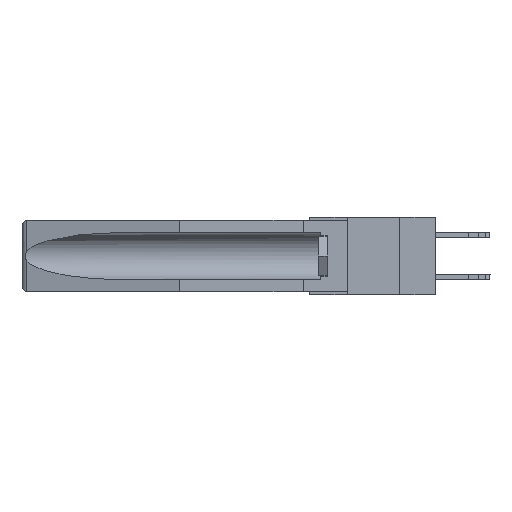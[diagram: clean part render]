
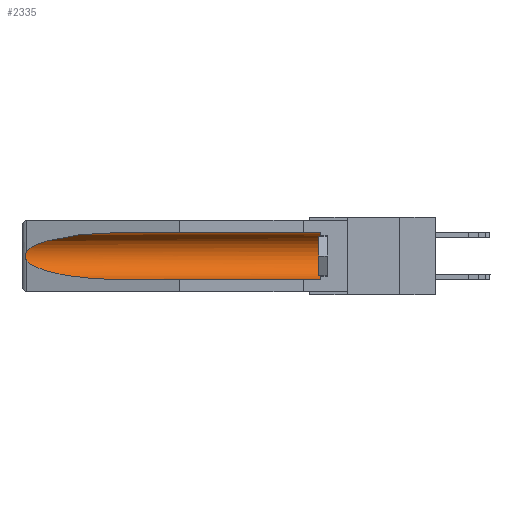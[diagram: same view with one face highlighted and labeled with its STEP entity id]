
A CAD part, left-side view. The second image highlights one B-rep face of the part: STEP entity #2335.
In plain terms, the highlighted cylindrical face has radius 2.857 mm (diameter 5.715 mm), a partial arc.
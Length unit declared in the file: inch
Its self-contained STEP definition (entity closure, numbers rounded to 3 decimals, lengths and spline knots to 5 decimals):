
#294 = VERTEX_POINT ( 'NONE', #1117 ) ;
#654 = CARTESIAN_POINT ( 'NONE',  ( 0.155, -0.30754, -0.059 ) ) ;
#737 = CARTESIAN_POINT ( 'NONE',  ( 0.2675, 1.53308, -0.17534 ) ) ;
#1117 = CARTESIAN_POINT ( 'NONE',  ( 0.155, 0.126, -0.059 ) ) ;
#1808 = EDGE_LOOP ( 'NONE', ( #21762, #15099, #2804, #14312, #2359, #7860 ) ) ;
#1947 = EDGE_CURVE ( 'NONE', #17766, #7095, #24393, .T. ) ;
#2003 = DIRECTION ( 'NONE',  ( 0., 1., 0. ) ) ;
#2260 = VECTOR ( 'NONE', #2003, 39.37008 ) ;
#2335 = ADVANCED_FACE ( 'NONE', ( #23821 ), #7049, .F. ) ;
#2359 = ORIENTED_EDGE ( 'NONE', *, *, #15660, .T. ) ;
#2804 = ORIENTED_EDGE ( 'NONE', *, *, #15588, .T. ) ;
#2831 = CARTESIAN_POINT ( 'NONE',  ( 0.26655, 1.53094, -0.18657 ) ) ;
#3069 = CARTESIAN_POINT ( 'NONE',  ( 0.155, 1.07973, -0.284 ) ) ;
#3543 = EDGE_CURVE ( 'NONE', #20831, #22787, #14787, .T. ) ;
#3709 = LINE ( 'NONE', #654, #21369 ) ;
#4520 = CARTESIAN_POINT ( 'NONE',  ( 0.2673, 1.5327, -0.16383 ) ) ;
#4676 = CARTESIAN_POINT ( 'NONE',  ( 0.26597, 1.52961, -0.15275 ) ) ;
#5734 = CARTESIAN_POINT ( 'NONE',  ( 0.155, -0.30754, -0.284 ) ) ;
#5834 = CARTESIAN_POINT ( 'NONE',  ( 0.155, 1.07973, -0.284 ) ) ;
#6392 = CARTESIAN_POINT ( 'NONE',  ( 0.2675, 1.53308, -0.16763 ) ) ;
#6776 = AXIS2_PLACEMENT_3D ( 'NONE', #16820, #13344, #22556 ) ;
#7049 = CYLINDRICAL_SURFACE ( 'NONE', #6776, 0.1125 ) ;
#7095 = VERTEX_POINT ( 'NONE', #17010 ) ;
#7124 = CIRCLE ( 'NONE', #22834, 0.1125 ) ;
#7848 = CARTESIAN_POINT ( 'NONE',  ( 0.25451, 1.48313, -0.24835 ) ) ;
#7860 = ORIENTED_EDGE ( 'NONE', *, *, #18494, .T. ) ;
#9028 = CARTESIAN_POINT ( 'NONE',  ( 0.26537, 1.52718, -0.14972 ) ) ;
#9183 = CARTESIAN_POINT ( 'NONE',  ( 0.155, 0.126, -0.284 ) ) ;
#9941 = CARTESIAN_POINT ( 'NONE',  ( 0.26537, 1.52718, -0.19328 ) ) ;
#10109 = DIRECTION ( 'NONE',  ( 0., -1., 0. ) ) ;
#10359 = CARTESIAN_POINT ( 'NONE',  ( 0.26597, 1.5296, -0.19026 ) ) ;
#11109 =( BOUNDED_CURVE ( )  B_SPLINE_CURVE ( 3, ( #9941, #7848, #17301, #5834 ),
 .UNSPECIFIED., .F., .F. ) 
 B_SPLINE_CURVE_WITH_KNOTS ( ( 4, 4 ),
 ( 0.1948, 1.5708 ),
 .UNSPECIFIED. ) 
 CURVE ( )  GEOMETRIC_REPRESENTATION_ITEM ( )  RATIONAL_B_SPLINE_CURVE ( ( 1., 0.848, 0.848, 1. ) ) 
 REPRESENTATION_ITEM ( '' )  );
#11907 =( BOUNDED_CURVE ( )  B_SPLINE_CURVE ( 3, ( #20336, #12751, #24069, #9028 ),
 .UNSPECIFIED., .F., .F. ) 
 B_SPLINE_CURVE_WITH_KNOTS ( ( 4, 4 ),
 ( 4.71239, 6.08839 ),
 .UNSPECIFIED. ) 
 CURVE ( )  GEOMETRIC_REPRESENTATION_ITEM ( )  RATIONAL_B_SPLINE_CURVE ( ( 1., 0.848, 0.848, 1. ) ) 
 REPRESENTATION_ITEM ( '' )  );
#12151 = CARTESIAN_POINT ( 'NONE',  ( 0.26537, 1.52718, -0.14972 ) ) ;
#12308 = CARTESIAN_POINT ( 'NONE',  ( 0.155, 0.126, -0.1715 ) ) ;
#12751 = CARTESIAN_POINT ( 'NONE',  ( 0.21114, 1.30732, -0.059 ) ) ;
#13344 = DIRECTION ( 'NONE',  ( 0., 1., 0. ) ) ;
#14312 = ORIENTED_EDGE ( 'NONE', *, *, #3543, .F. ) ;
#14787 = LINE ( 'NONE', #5734, #2260 ) ;
#15099 = ORIENTED_EDGE ( 'NONE', *, *, #1947, .T. ) ;
#15588 = EDGE_CURVE ( 'NONE', #7095, #22787, #11109, .T. ) ;
#15660 = EDGE_CURVE ( 'NONE', #20831, #294, #7124, .T. ) ;
#16472 = CARTESIAN_POINT ( 'NONE',  ( 0.26537, 1.52718, -0.14972 ) ) ;
#16820 = CARTESIAN_POINT ( 'NONE',  ( 0.155, -0.30754, -0.1715 ) ) ;
#17010 = CARTESIAN_POINT ( 'NONE',  ( 0.26537, 1.52718, -0.19328 ) ) ;
#17142 = CARTESIAN_POINT ( 'NONE',  ( 0.155, 1.07973, -0.059 ) ) ;
#17301 = CARTESIAN_POINT ( 'NONE',  ( 0.21114, 1.30732, -0.284 ) ) ;
#17766 = VERTEX_POINT ( 'NONE', #16472 ) ;
#17774 = DIRECTION ( 'NONE',  ( 0., 0., 1. ) ) ;
#18494 = EDGE_CURVE ( 'NONE', #294, #21883, #3709, .T. ) ;
#19868 = CARTESIAN_POINT ( 'NONE',  ( 0.2673, 1.53269, -0.17917 ) ) ;
#20038 = CARTESIAN_POINT ( 'NONE',  ( 0.26654, 1.53092, -0.15636 ) ) ;
#20336 = CARTESIAN_POINT ( 'NONE',  ( 0.155, 1.07973, -0.059 ) ) ;
#20831 = VERTEX_POINT ( 'NONE', #9183 ) ;
#21238 = EDGE_CURVE ( 'NONE', #21883, #17766, #11907, .T. ) ;
#21369 = VECTOR ( 'NONE', #21401, 39.37008 ) ;
#21401 = DIRECTION ( 'NONE',  ( 0., 1., 0. ) ) ;
#21762 = ORIENTED_EDGE ( 'NONE', *, *, #21238, .T. ) ;
#21883 = VERTEX_POINT ( 'NONE', #17142 ) ;
#21959 = CARTESIAN_POINT ( 'NONE',  ( 0.26537, 1.52718, -0.19328 ) ) ;
#22556 = DIRECTION ( 'NONE',  ( 0., 0., 1. ) ) ;
#22787 = VERTEX_POINT ( 'NONE', #3069 ) ;
#22834 = AXIS2_PLACEMENT_3D ( 'NONE', #12308, #10109, #17774 ) ;
#23821 = FACE_OUTER_BOUND ( 'NONE', #1808, .T. ) ;
#24069 = CARTESIAN_POINT ( 'NONE',  ( 0.25451, 1.48313, -0.09465 ) ) ;
#24393 = B_SPLINE_CURVE_WITH_KNOTS ( 'NONE', 3,
 ( #12151, #4676, #20038, #4520, #6392, #737, #19868, #2831, #10359, #21959 ),
 .UNSPECIFIED., .F., .F.,
 ( 4, 2, 2, 2, 4 ),
 ( 0., 0.00029, 0.00058, 0.00087, 0.00117 ),
 .UNSPECIFIED. ) ;
